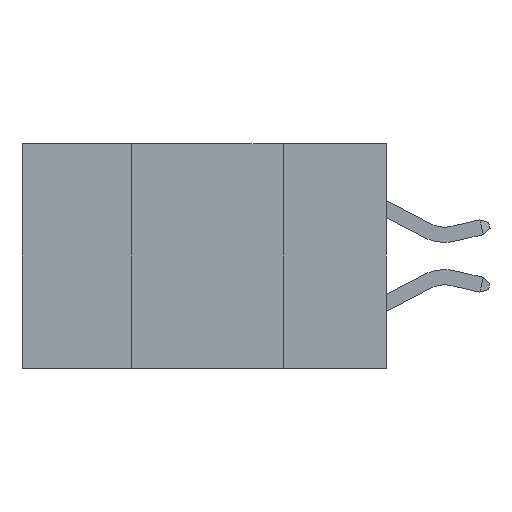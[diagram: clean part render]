
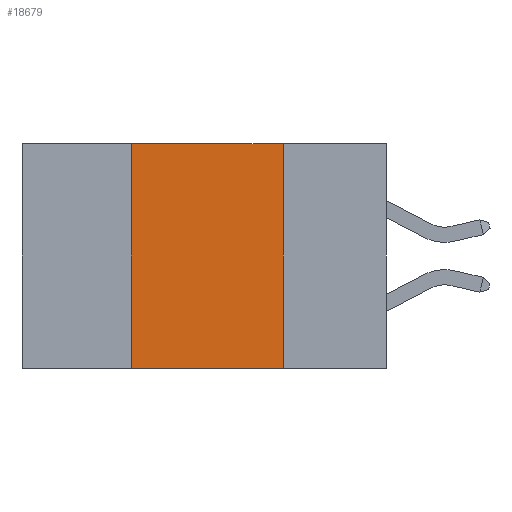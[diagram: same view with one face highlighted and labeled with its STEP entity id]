
A CAD part, left-side view. The second image highlights one B-rep face of the part: STEP entity #18679.
In plain terms, the highlighted planar face has unit normal (-1, 0, 0).
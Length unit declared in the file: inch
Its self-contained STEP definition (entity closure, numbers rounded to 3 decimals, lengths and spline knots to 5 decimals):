
#225 = DIRECTION ( 'NONE',  ( 0., 0., 1. ) ) ;
#378 = DIRECTION ( 'NONE',  ( 1., 0., 0. ) ) ;
#1625 = FACE_OUTER_BOUND ( 'NONE', #18926, .T. ) ;
#3096 = CARTESIAN_POINT ( 'NONE',  ( 0., 0.42, 0. ) ) ;
#3862 = ORIENTED_EDGE ( 'NONE', *, *, #27601, .F. ) ;
#4026 = VECTOR ( 'NONE', #4406, 39.37008 ) ;
#4406 = DIRECTION ( 'NONE',  ( 0., 0., -1. ) ) ;
#5272 = DIRECTION ( 'NONE',  ( 0., -1., 0. ) ) ;
#7470 = VECTOR ( 'NONE', #32738, 39.37008 ) ;
#8093 = CARTESIAN_POINT ( 'NONE',  ( 0., 0.42, 0. ) ) ;
#9492 = CARTESIAN_POINT ( 'NONE',  ( 0., 0.17, 0. ) ) ;
#10373 = CARTESIAN_POINT ( 'NONE',  ( 0., 0.6, 0. ) ) ;
#10450 = VECTOR ( 'NONE', #225, 39.37008 ) ;
#11233 = EDGE_CURVE ( 'NONE', #28995, #17103, #14370, .T. ) ;
#13800 = AXIS2_PLACEMENT_3D ( 'NONE', #21061, #378, #18581 ) ;
#14370 = LINE ( 'NONE', #22484, #7470 ) ;
#17103 = VERTEX_POINT ( 'NONE', #28821 ) ;
#18003 = VERTEX_POINT ( 'NONE', #3096 ) ;
#18581 = DIRECTION ( 'NONE',  ( 0., 0., -1. ) ) ;
#18626 = LINE ( 'NONE', #9492, #4026 ) ;
#18679 = ADVANCED_FACE ( 'NONE', ( #1625 ), #28796, .F. ) ;
#18926 = EDGE_LOOP ( 'NONE', ( #23714, #3862, #25330, #32106 ) ) ;
#18989 = VECTOR ( 'NONE', #5272, 39.37008 ) ;
#19057 = EDGE_CURVE ( 'NONE', #24623, #17103, #18626, .T. ) ;
#21061 = CARTESIAN_POINT ( 'NONE',  ( 0., 0.6, 0. ) ) ;
#22484 = CARTESIAN_POINT ( 'NONE',  ( 0., 0.6, -0.37 ) ) ;
#23714 = ORIENTED_EDGE ( 'NONE', *, *, #19057, .F. ) ;
#24623 = VERTEX_POINT ( 'NONE', #28075 ) ;
#25330 = ORIENTED_EDGE ( 'NONE', *, *, #27671, .F. ) ;
#26196 = CARTESIAN_POINT ( 'NONE',  ( 0., 0.42, -0.37 ) ) ;
#27601 = EDGE_CURVE ( 'NONE', #18003, #24623, #32622, .T. ) ;
#27671 = EDGE_CURVE ( 'NONE', #28995, #18003, #31811, .T. ) ;
#28075 = CARTESIAN_POINT ( 'NONE',  ( 0., 0.17, 0. ) ) ;
#28796 = PLANE ( 'NONE',  #13800 ) ;
#28821 = CARTESIAN_POINT ( 'NONE',  ( 0., 0.17, -0.37 ) ) ;
#28995 = VERTEX_POINT ( 'NONE', #26196 ) ;
#31811 = LINE ( 'NONE', #8093, #10450 ) ;
#32106 = ORIENTED_EDGE ( 'NONE', *, *, #11233, .T. ) ;
#32622 = LINE ( 'NONE', #10373, #18989 ) ;
#32738 = DIRECTION ( 'NONE',  ( 0., -1., 0. ) ) ;
